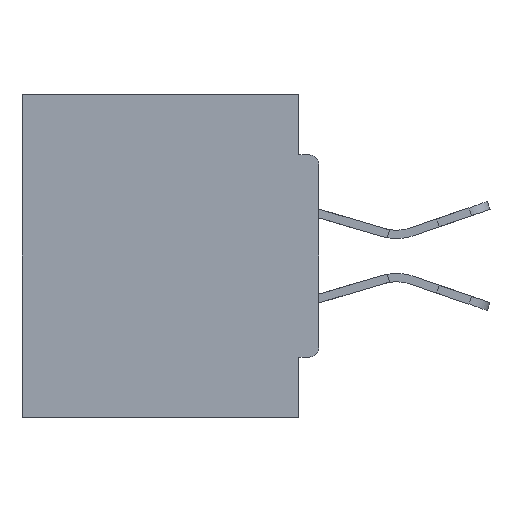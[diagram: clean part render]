
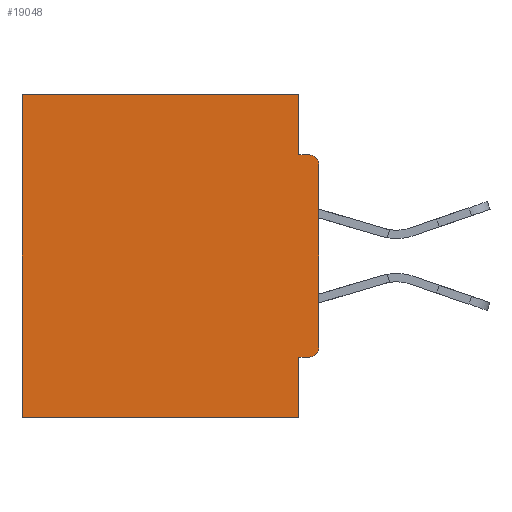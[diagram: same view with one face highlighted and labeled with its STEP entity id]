
A CAD part, left-side view. The second image highlights one B-rep face of the part: STEP entity #19048.
In plain terms, the highlighted planar face has unit normal (-1, 0, 0).
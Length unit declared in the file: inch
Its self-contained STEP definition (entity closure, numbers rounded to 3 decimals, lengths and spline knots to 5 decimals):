
#580 = DIRECTION ( 'NONE',  ( 0., 0., -1. ) ) ;
#614 = DIRECTION ( 'NONE',  ( 1., 0., 0. ) ) ;
#1333 = VECTOR ( 'NONE', #23255, 39.37008 ) ;
#1473 = VERTEX_POINT ( 'NONE', #34768 ) ;
#1810 = VERTEX_POINT ( 'NONE', #34294 ) ;
#1906 = CARTESIAN_POINT ( 'NONE',  ( 0.298, 0.46, 0. ) ) ;
#1988 = AXIS2_PLACEMENT_3D ( 'NONE', #24214, #614, #30472 ) ;
#3142 = CARTESIAN_POINT ( 'NONE',  ( 0.298, 0.46, 0. ) ) ;
#3302 = CARTESIAN_POINT ( 'NONE',  ( 0.298, 0.015, -0.4065 ) ) ;
#3733 = CARTESIAN_POINT ( 'NONE',  ( 0.298, 0., 0. ) ) ;
#3934 = EDGE_CURVE ( 'NONE', #25857, #32485, #30162, .T. ) ;
#4016 = DIRECTION ( 'NONE',  ( 0., 0., -1. ) ) ;
#4252 = CIRCLE ( 'NONE', #9967, 0.015 ) ;
#5094 = VECTOR ( 'NONE', #20700, 39.37008 ) ;
#6088 = DIRECTION ( 'NONE',  ( 0., 1., 0. ) ) ;
#7437 = LINE ( 'NONE', #1906, #1333 ) ;
#7443 = CARTESIAN_POINT ( 'NONE',  ( 0.298, 0.031, -0.5 ) ) ;
#8067 = CARTESIAN_POINT ( 'NONE',  ( 0.298, 0., -0.1085 ) ) ;
#8216 = CARTESIAN_POINT ( 'NONE',  ( 0.298, 0.031, -0.5 ) ) ;
#8249 = LINE ( 'NONE', #37581, #26239 ) ;
#8566 = ORIENTED_EDGE ( 'NONE', *, *, #26049, .T. ) ;
#8693 = CIRCLE ( 'NONE', #17964, 0.015 ) ;
#9267 = CARTESIAN_POINT ( 'NONE',  ( 0.298, 0.015, -0.1085 ) ) ;
#9374 = LINE ( 'NONE', #31108, #23535 ) ;
#9967 = AXIS2_PLACEMENT_3D ( 'NONE', #9267, #18353, #580 ) ;
#10197 = CARTESIAN_POINT ( 'NONE',  ( 0.298, 0.031, 0. ) ) ;
#10691 = VERTEX_POINT ( 'NONE', #3302 ) ;
#10710 = CARTESIAN_POINT ( 'NONE',  ( 0.298, 0., -0.3915 ) ) ;
#11154 = DIRECTION ( 'NONE',  ( 0., 0., -1. ) ) ;
#11168 = ORIENTED_EDGE ( 'NONE', *, *, #16032, .F. ) ;
#11252 = EDGE_CURVE ( 'NONE', #21635, #38780, #9374, .T. ) ;
#11285 = CARTESIAN_POINT ( 'NONE',  ( 0.298, 0.46, -0.5 ) ) ;
#11288 = DIRECTION ( 'NONE',  ( -1., 0., 0. ) ) ;
#11704 = EDGE_CURVE ( 'NONE', #10691, #21635, #31105, .T. ) ;
#13884 = CARTESIAN_POINT ( 'NONE',  ( 0.298, 0.015, -0.3915 ) ) ;
#14266 = ORIENTED_EDGE ( 'NONE', *, *, #11704, .F. ) ;
#15007 = EDGE_LOOP ( 'NONE', ( #8566, #20533, #38298, #38820, #19813, #11168, #38694, #14266, #17453, #38784 ) ) ;
#15220 = PLANE ( 'NONE',  #1988 ) ;
#16032 = EDGE_CURVE ( 'NONE', #38780, #17481, #29506, .T. ) ;
#17453 = ORIENTED_EDGE ( 'NONE', *, *, #22188, .T. ) ;
#17481 = VERTEX_POINT ( 'NONE', #11285 ) ;
#17964 = AXIS2_PLACEMENT_3D ( 'NONE', #13884, #11288, #11154 ) ;
#18353 = DIRECTION ( 'NONE',  ( -1., 0., 0. ) ) ;
#18469 = LINE ( 'NONE', #8216, #23225 ) ;
#19048 = ADVANCED_FACE ( 'NONE', ( #34922 ), #15220, .F. ) ;
#19382 = EDGE_CURVE ( 'NONE', #32485, #17481, #7437, .T. ) ;
#19813 = ORIENTED_EDGE ( 'NONE', *, *, #19382, .T. ) ;
#20533 = ORIENTED_EDGE ( 'NONE', *, *, #21558, .F. ) ;
#20700 = DIRECTION ( 'NONE',  ( 0., 1., 0. ) ) ;
#21558 = EDGE_CURVE ( 'NONE', #1473, #1810, #8249, .T. ) ;
#21635 = VERTEX_POINT ( 'NONE', #31921 ) ;
#22188 = EDGE_CURVE ( 'NONE', #10691, #35678, #8693, .T. ) ;
#22636 = DIRECTION ( 'NONE',  ( 0., -1., 0. ) ) ;
#23225 = VECTOR ( 'NONE', #35199, 39.37008 ) ;
#23255 = DIRECTION ( 'NONE',  ( 0., 0., -1. ) ) ;
#23535 = VECTOR ( 'NONE', #4016, 39.37008 ) ;
#24214 = CARTESIAN_POINT ( 'NONE',  ( 0.298, 0., 0. ) ) ;
#24232 = DIRECTION ( 'NONE',  ( 0., 1., 0. ) ) ;
#24969 = DIRECTION ( 'NONE',  ( 0., 0., -1. ) ) ;
#25857 = VERTEX_POINT ( 'NONE', #10197 ) ;
#26049 = EDGE_CURVE ( 'NONE', #31317, #1810, #4252, .T. ) ;
#26183 = VECTOR ( 'NONE', #6088, 39.37008 ) ;
#26239 = VECTOR ( 'NONE', #22636, 39.37008 ) ;
#29506 = LINE ( 'NONE', #36323, #26183 ) ;
#30162 = LINE ( 'NONE', #32853, #37200 ) ;
#30472 = DIRECTION ( 'NONE',  ( 0., 0., -1. ) ) ;
#31105 = LINE ( 'NONE', #32749, #5094 ) ;
#31108 = CARTESIAN_POINT ( 'NONE',  ( 0.298, 0.031, -0.5 ) ) ;
#31317 = VERTEX_POINT ( 'NONE', #8067 ) ;
#31921 = CARTESIAN_POINT ( 'NONE',  ( 0.298, 0.031, -0.4065 ) ) ;
#32485 = VERTEX_POINT ( 'NONE', #3142 ) ;
#32749 = CARTESIAN_POINT ( 'NONE',  ( 0.298, 0., -0.4065 ) ) ;
#32853 = CARTESIAN_POINT ( 'NONE',  ( 0.298, 0., 0. ) ) ;
#33886 = LINE ( 'NONE', #3733, #36216 ) ;
#34052 = EDGE_CURVE ( 'NONE', #31317, #35678, #33886, .T. ) ;
#34294 = CARTESIAN_POINT ( 'NONE',  ( 0.298, 0.015, -0.0935 ) ) ;
#34768 = CARTESIAN_POINT ( 'NONE',  ( 0.298, 0.031, -0.0935 ) ) ;
#34922 = FACE_OUTER_BOUND ( 'NONE', #15007, .T. ) ;
#35199 = DIRECTION ( 'NONE',  ( 0., 0., -1. ) ) ;
#35678 = VERTEX_POINT ( 'NONE', #10710 ) ;
#36216 = VECTOR ( 'NONE', #24969, 39.37008 ) ;
#36323 = CARTESIAN_POINT ( 'NONE',  ( 0.298, 0., -0.5 ) ) ;
#36863 = EDGE_CURVE ( 'NONE', #25857, #1473, #18469, .T. ) ;
#37200 = VECTOR ( 'NONE', #24232, 39.37008 ) ;
#37581 = CARTESIAN_POINT ( 'NONE',  ( 0.298, 0., -0.0935 ) ) ;
#38298 = ORIENTED_EDGE ( 'NONE', *, *, #36863, .F. ) ;
#38694 = ORIENTED_EDGE ( 'NONE', *, *, #11252, .F. ) ;
#38780 = VERTEX_POINT ( 'NONE', #7443 ) ;
#38784 = ORIENTED_EDGE ( 'NONE', *, *, #34052, .F. ) ;
#38820 = ORIENTED_EDGE ( 'NONE', *, *, #3934, .T. ) ;
